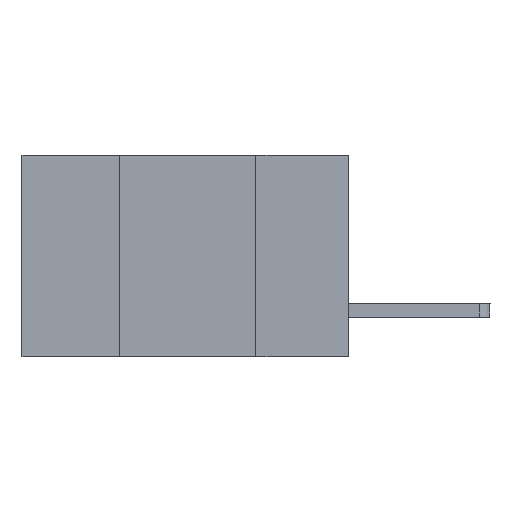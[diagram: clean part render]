
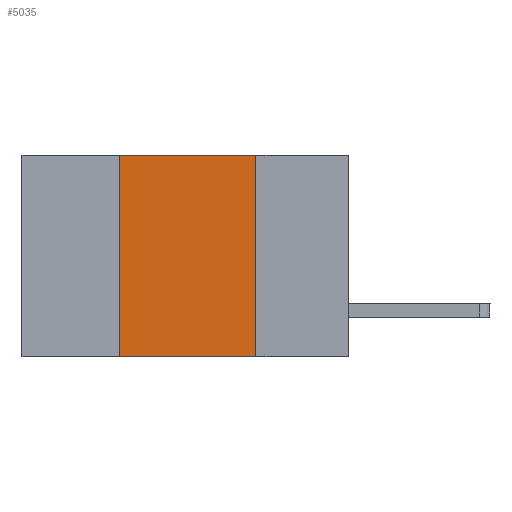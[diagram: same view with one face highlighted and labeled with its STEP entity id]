
A CAD part, left-side view. The second image highlights one B-rep face of the part: STEP entity #5035.
In plain terms, the highlighted planar face has unit normal (-1, 0, 0).
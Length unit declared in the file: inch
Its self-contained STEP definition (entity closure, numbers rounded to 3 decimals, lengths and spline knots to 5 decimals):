
#45 = FACE_OUTER_BOUND ( 'NONE', #5180, .T. ) ;
#277 = DIRECTION ( 'NONE',  ( 0., -1., 0. ) ) ;
#571 = LINE ( 'NONE', #3900, #1415 ) ;
#679 = CARTESIAN_POINT ( 'NONE',  ( 0., 0.17, 0. ) ) ;
#765 = ORIENTED_EDGE ( 'NONE', *, *, #4418, .F. ) ;
#836 = LINE ( 'NONE', #10013, #10655 ) ;
#933 = VECTOR ( 'NONE', #5040, 39.37008 ) ;
#984 = VERTEX_POINT ( 'NONE', #6973 ) ;
#1415 = VECTOR ( 'NONE', #3978, 39.37008 ) ;
#2458 = VERTEX_POINT ( 'NONE', #6739 ) ;
#2550 = VECTOR ( 'NONE', #277, 39.37008 ) ;
#3276 = PLANE ( 'NONE',  #4623 ) ;
#3406 = CARTESIAN_POINT ( 'NONE',  ( 0., 0.6, -0.37 ) ) ;
#3891 = ORIENTED_EDGE ( 'NONE', *, *, #5556, .T. ) ;
#3900 = CARTESIAN_POINT ( 'NONE',  ( 0., 0.17, 0. ) ) ;
#3978 = DIRECTION ( 'NONE',  ( 0., 0., -1. ) ) ;
#4418 = EDGE_CURVE ( 'NONE', #7877, #9451, #836, .T. ) ;
#4623 = AXIS2_PLACEMENT_3D ( 'NONE', #10645, #8944, #10685 ) ;
#5027 = ORIENTED_EDGE ( 'NONE', *, *, #7514, .F. ) ;
#5035 = ADVANCED_FACE ( 'NONE', ( #45 ), #3276, .F. ) ;
#5040 = DIRECTION ( 'NONE',  ( 0., 0., 1. ) ) ;
#5180 = EDGE_LOOP ( 'NONE', ( #5027, #765, #5272, #3891 ) ) ;
#5272 = ORIENTED_EDGE ( 'NONE', *, *, #11365, .F. ) ;
#5556 = EDGE_CURVE ( 'NONE', #2458, #984, #6346, .T. ) ;
#5704 = LINE ( 'NONE', #7293, #933 ) ;
#6346 = LINE ( 'NONE', #3406, #2550 ) ;
#6739 = CARTESIAN_POINT ( 'NONE',  ( 0., 0.42, -0.37 ) ) ;
#6973 = CARTESIAN_POINT ( 'NONE',  ( 0., 0.17, -0.37 ) ) ;
#7256 = CARTESIAN_POINT ( 'NONE',  ( 0., 0.42, 0. ) ) ;
#7293 = CARTESIAN_POINT ( 'NONE',  ( 0., 0.42, 0. ) ) ;
#7514 = EDGE_CURVE ( 'NONE', #9451, #984, #571, .T. ) ;
#7877 = VERTEX_POINT ( 'NONE', #7256 ) ;
#8944 = DIRECTION ( 'NONE',  ( 1., 0., 0. ) ) ;
#9451 = VERTEX_POINT ( 'NONE', #679 ) ;
#10013 = CARTESIAN_POINT ( 'NONE',  ( 0., 0.6, 0. ) ) ;
#10645 = CARTESIAN_POINT ( 'NONE',  ( 0., 0.6, 0. ) ) ;
#10655 = VECTOR ( 'NONE', #10887, 39.37008 ) ;
#10685 = DIRECTION ( 'NONE',  ( 0., 0., -1. ) ) ;
#10887 = DIRECTION ( 'NONE',  ( 0., -1., 0. ) ) ;
#11365 = EDGE_CURVE ( 'NONE', #2458, #7877, #5704, .T. ) ;
